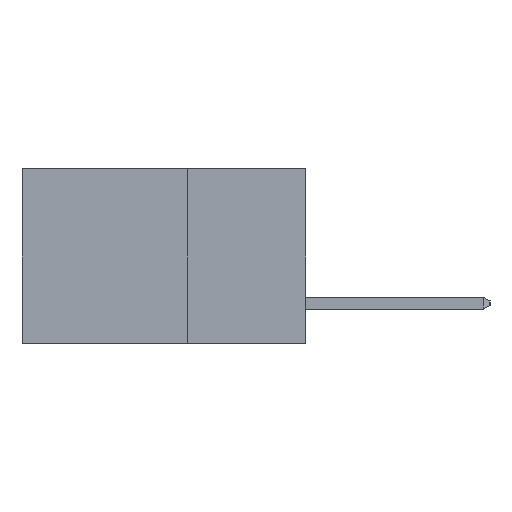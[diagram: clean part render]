
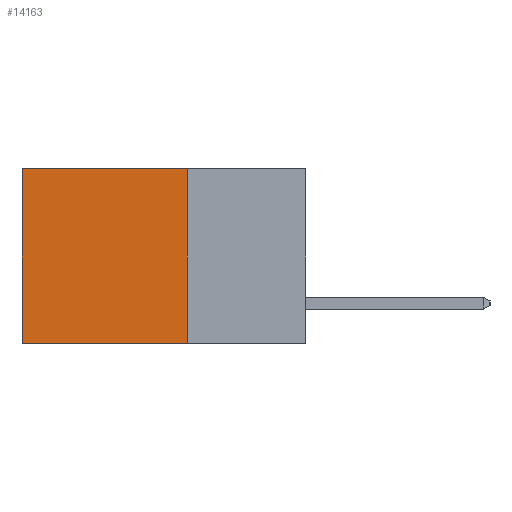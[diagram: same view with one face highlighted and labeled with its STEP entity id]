
A CAD part, left-side view. The second image highlights one B-rep face of the part: STEP entity #14163.
In plain terms, the highlighted planar face has unit normal (-1, 0, 0).
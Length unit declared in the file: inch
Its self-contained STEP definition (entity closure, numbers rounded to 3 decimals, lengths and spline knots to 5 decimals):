
#628 = LINE ( 'NONE', #3182, #1091 ) ;
#1045 = EDGE_CURVE ( 'NONE', #3932, #9197, #18212, .T. ) ;
#1091 = VECTOR ( 'NONE', #4666, 39.37008 ) ;
#2750 = VECTOR ( 'NONE', #8177, 39.37008 ) ;
#3182 = CARTESIAN_POINT ( 'NONE',  ( 0.2615, 0.6, -0.37 ) ) ;
#3932 = VERTEX_POINT ( 'NONE', #14333 ) ;
#4666 = DIRECTION ( 'NONE',  ( 0., 0., -1. ) ) ;
#5655 = DIRECTION ( 'NONE',  ( 0., 1., 0. ) ) ;
#5684 = ORIENTED_EDGE ( 'NONE', *, *, #8806, .F. ) ;
#7124 = VECTOR ( 'NONE', #8852, 39.37008 ) ;
#7125 = ORIENTED_EDGE ( 'NONE', *, *, #15818, .T. ) ;
#7265 = DIRECTION ( 'NONE',  ( 0., 0., -1. ) ) ;
#7287 = DIRECTION ( 'NONE',  ( 1., 0., 0. ) ) ;
#7337 = CARTESIAN_POINT ( 'NONE',  ( 0.2615, 0.25, -0.37 ) ) ;
#7445 = PLANE ( 'NONE',  #13003 ) ;
#8018 = CARTESIAN_POINT ( 'NONE',  ( 0.2615, 0.25, 0. ) ) ;
#8177 = DIRECTION ( 'NONE',  ( 0., 0., -1. ) ) ;
#8382 = VERTEX_POINT ( 'NONE', #9571 ) ;
#8453 = CARTESIAN_POINT ( 'NONE',  ( 0.2615, 0.25, -0.37 ) ) ;
#8591 = ORIENTED_EDGE ( 'NONE', *, *, #15052, .F. ) ;
#8806 = EDGE_CURVE ( 'NONE', #3932, #8382, #9703, .T. ) ;
#8852 = DIRECTION ( 'NONE',  ( 0., 1., 0. ) ) ;
#9197 = VERTEX_POINT ( 'NONE', #14369 ) ;
#9571 = CARTESIAN_POINT ( 'NONE',  ( 0.2615, 0.25, -0.37 ) ) ;
#9703 = LINE ( 'NONE', #8453, #2750 ) ;
#10043 = VECTOR ( 'NONE', #5655, 39.37008 ) ;
#11266 = FACE_OUTER_BOUND ( 'NONE', #17297, .T. ) ;
#11495 = LINE ( 'NONE', #15866, #7124 ) ;
#13003 = AXIS2_PLACEMENT_3D ( 'NONE', #7337, #7287, #7265 ) ;
#13242 = VERTEX_POINT ( 'NONE', #15107 ) ;
#14163 = ADVANCED_FACE ( 'NONE', ( #11266 ), #7445, .F. ) ;
#14333 = CARTESIAN_POINT ( 'NONE',  ( 0.2615, 0.25, 0. ) ) ;
#14369 = CARTESIAN_POINT ( 'NONE',  ( 0.2615, 0.6, 0. ) ) ;
#15052 = EDGE_CURVE ( 'NONE', #8382, #13242, #11495, .T. ) ;
#15107 = CARTESIAN_POINT ( 'NONE',  ( 0.2615, 0.6, -0.37 ) ) ;
#15818 = EDGE_CURVE ( 'NONE', #9197, #13242, #628, .T. ) ;
#15866 = CARTESIAN_POINT ( 'NONE',  ( 0.2615, 0.25, -0.37 ) ) ;
#16729 = ORIENTED_EDGE ( 'NONE', *, *, #1045, .T. ) ;
#17297 = EDGE_LOOP ( 'NONE', ( #7125, #8591, #5684, #16729 ) ) ;
#18212 = LINE ( 'NONE', #8018, #10043 ) ;
